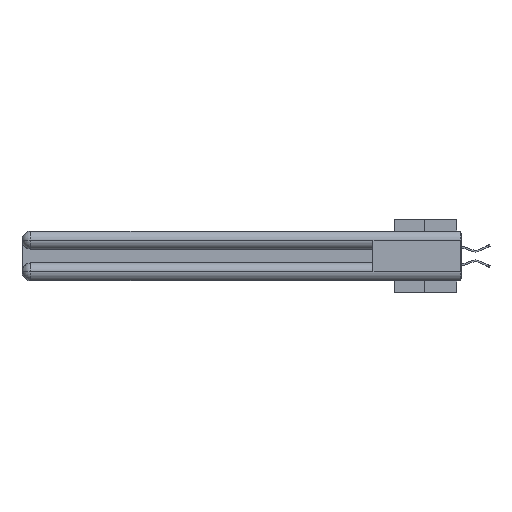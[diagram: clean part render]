
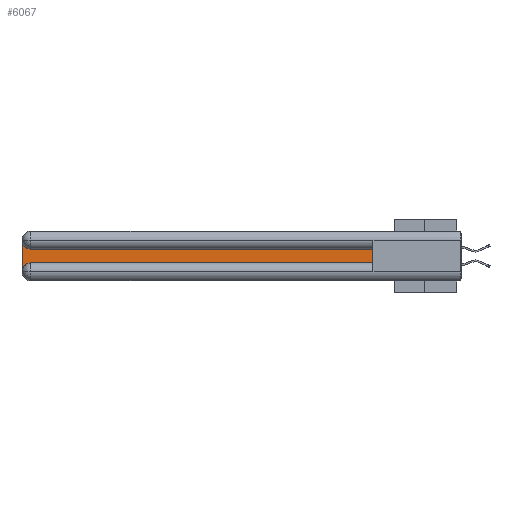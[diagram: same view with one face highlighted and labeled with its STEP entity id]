
A CAD part, left-side view. The second image highlights one B-rep face of the part: STEP entity #6067.
In plain terms, the highlighted planar face has unit normal (-1, 0, 0).
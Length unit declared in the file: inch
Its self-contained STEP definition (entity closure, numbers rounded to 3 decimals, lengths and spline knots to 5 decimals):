
#324 = LINE ( 'NONE', #8029, #25573 ) ;
#1022 = EDGE_CURVE ( 'NONE', #16608, #30951, #30597, .T. ) ;
#2630 = VERTEX_POINT ( 'NONE', #11625 ) ;
#2747 = AXIS2_PLACEMENT_3D ( 'NONE', #34118, #13721, #6366 ) ;
#5375 = DIRECTION ( 'NONE',  ( 1., 0., 0. ) ) ;
#6067 = ADVANCED_FACE ( 'NONE', ( #18254 ), #13134, .F. ) ;
#6366 = DIRECTION ( 'NONE',  ( 0., 0., -1. ) ) ;
#6695 = CARTESIAN_POINT ( 'NONE',  ( 0.075, 2.94, -0.1225 ) ) ;
#7136 = ORIENTED_EDGE ( 'NONE', *, *, #9008, .T. ) ;
#7749 = LINE ( 'NONE', #21697, #37782 ) ;
#8029 = CARTESIAN_POINT ( 'NONE',  ( 0.075, 0.6, -0.2175 ) ) ;
#9008 = EDGE_CURVE ( 'NONE', #35825, #16608, #15984, .T. ) ;
#9818 = VERTEX_POINT ( 'NONE', #10703 ) ;
#10703 = CARTESIAN_POINT ( 'NONE',  ( 0.075, 2.94, -0.2175 ) ) ;
#11625 = CARTESIAN_POINT ( 'NONE',  ( 0.075, 0.6, -0.2175 ) ) ;
#12989 = EDGE_LOOP ( 'NONE', ( #7136, #23768, #22490, #26048, #37970, #41340 ) ) ;
#13134 = PLANE ( 'NONE',  #2747 ) ;
#13721 = DIRECTION ( 'NONE',  ( 1., 0., 0. ) ) ;
#15515 = DIRECTION ( 'NONE',  ( 0., 0., -1. ) ) ;
#15984 = LINE ( 'NONE', #21679, #19234 ) ;
#16608 = VERTEX_POINT ( 'NONE', #6695 ) ;
#18254 = FACE_OUTER_BOUND ( 'NONE', #12989, .T. ) ;
#18284 = CARTESIAN_POINT ( 'NONE',  ( 0.075, 2.94, -0.2775 ) ) ;
#18399 = DIRECTION ( 'NONE',  ( 0., -1., 0. ) ) ;
#19234 = VECTOR ( 'NONE', #21966, 39.37008 ) ;
#21679 = CARTESIAN_POINT ( 'NONE',  ( 0.075, 0.6, -0.1225 ) ) ;
#21697 = CARTESIAN_POINT ( 'NONE',  ( 0.075, 3., -0.2175 ) ) ;
#21966 = DIRECTION ( 'NONE',  ( 0., 1., 0. ) ) ;
#22238 = CARTESIAN_POINT ( 'NONE',  ( 0.075, 2.94, -0.0625 ) ) ;
#22490 = ORIENTED_EDGE ( 'NONE', *, *, #25176, .T. ) ;
#22821 = CARTESIAN_POINT ( 'NONE',  ( 0.075, 0.6, -0.2175 ) ) ;
#23768 = ORIENTED_EDGE ( 'NONE', *, *, #1022, .T. ) ;
#24749 = VECTOR ( 'NONE', #26409, 39.37008 ) ;
#25176 = EDGE_CURVE ( 'NONE', #30951, #41714, #7749, .T. ) ;
#25573 = VECTOR ( 'NONE', #18399, 39.37008 ) ;
#26048 = ORIENTED_EDGE ( 'NONE', *, *, #36644, .T. ) ;
#26409 = DIRECTION ( 'NONE',  ( 0., 0., 1. ) ) ;
#28013 = CARTESIAN_POINT ( 'NONE',  ( 0.075, 3., -0.2775 ) ) ;
#28471 = DIRECTION ( 'NONE',  ( 1., 0., 0. ) ) ;
#30597 = CIRCLE ( 'NONE', #37227, 0.06 ) ;
#30951 = VERTEX_POINT ( 'NONE', #41443 ) ;
#33125 = CIRCLE ( 'NONE', #42892, 0.06 ) ;
#34118 = CARTESIAN_POINT ( 'NONE',  ( 0.075, 3., -0.1225 ) ) ;
#35825 = VERTEX_POINT ( 'NONE', #43059 ) ;
#36644 = EDGE_CURVE ( 'NONE', #41714, #9818, #33125, .T. ) ;
#37227 = AXIS2_PLACEMENT_3D ( 'NONE', #22238, #5375, #39311 ) ;
#37782 = VECTOR ( 'NONE', #15515, 39.37008 ) ;
#37970 = ORIENTED_EDGE ( 'NONE', *, *, #38215, .T. ) ;
#38215 = EDGE_CURVE ( 'NONE', #9818, #2630, #324, .T. ) ;
#39311 = DIRECTION ( 'NONE',  ( 0., 0., -1. ) ) ;
#41340 = ORIENTED_EDGE ( 'NONE', *, *, #42811, .T. ) ;
#41443 = CARTESIAN_POINT ( 'NONE',  ( 0.075, 3., -0.0625 ) ) ;
#41705 = DIRECTION ( 'NONE',  ( 0., 0., -1. ) ) ;
#41714 = VERTEX_POINT ( 'NONE', #28013 ) ;
#42811 = EDGE_CURVE ( 'NONE', #2630, #35825, #43031, .T. ) ;
#42892 = AXIS2_PLACEMENT_3D ( 'NONE', #18284, #28471, #41705 ) ;
#43031 = LINE ( 'NONE', #22821, #24749 ) ;
#43059 = CARTESIAN_POINT ( 'NONE',  ( 0.075, 0.6, -0.1225 ) ) ;
